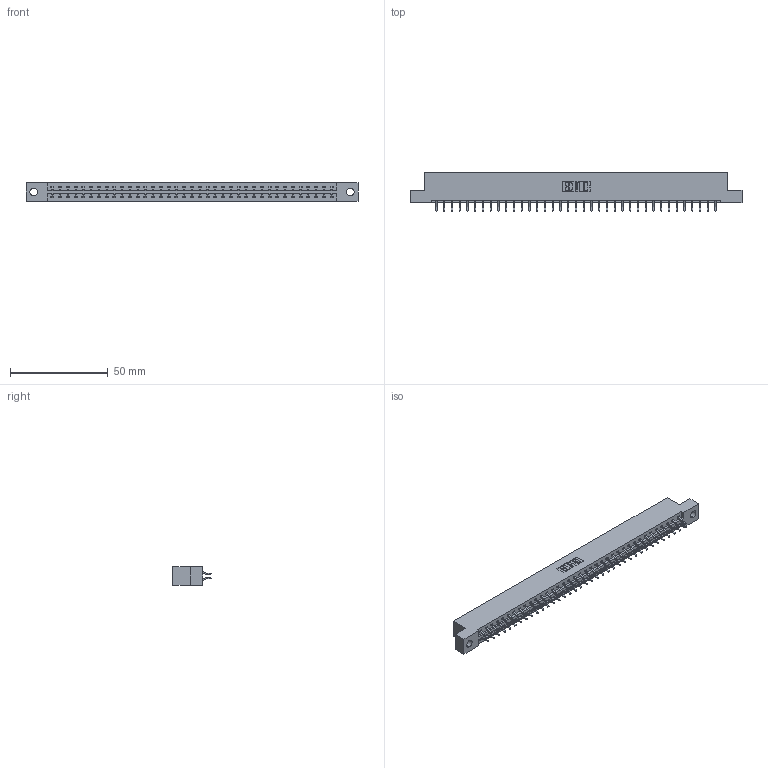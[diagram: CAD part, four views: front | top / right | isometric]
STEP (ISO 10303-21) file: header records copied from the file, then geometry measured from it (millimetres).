
FILE_DESCRIPTION (( 'STEP AP203' ), '1' );
FILE_NAME ('387-074-556-204.STEP', '2019-10-22T02:18:09', ( '' ), ( '' ), 'SwSTEP 2.0', 'SolidWorks 2016', '' );
FILE_SCHEMA (( 'CONFIG_CONTROL_DESIGN' ));
Length unit declared in the file: inch
Products named in the file (3): 345-292-001_556 Tail; 337 Part_Flush Mounting Lugs - 0.156 Dia-TH; 387-074-556-204
Assembly tree (75 placements, depth 2):
  387-074-556-204
    337 Part_Flush Mounting Lugs - 0.156 Dia-TH
    345-292-001_556 Tail  x74
Bounding box: 169.62 x 19.57 x 9.4 mm (x, y, z)
Volume: 17718.7 mm3; surface area: 19701.8 mm2
Topology: 75 solids, 75 shells, 4554 faces, 13557 edges, 8938 vertices
Faces by surface type: plane 3178, cylinder 1376
Entity records: 29557 total; most frequent: CARTESIAN_POINT 4998, ORIENTED_EDGE 4922, DIRECTION 4249, EDGE_CURVE 2461, LINE 2325, VECTOR 2325, VERTEX_POINT 1638, AXIS2_PLACEMENT_3D 962
